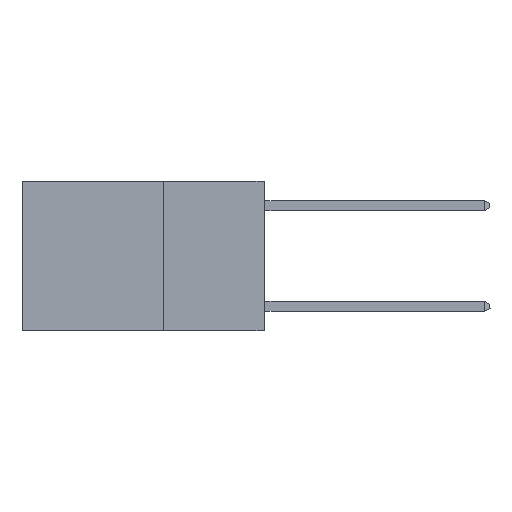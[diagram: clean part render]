
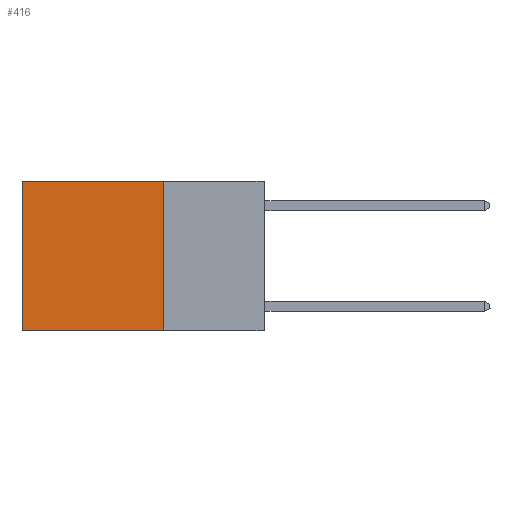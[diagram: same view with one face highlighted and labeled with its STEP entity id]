
A CAD part, left-side view. The second image highlights one B-rep face of the part: STEP entity #416.
In plain terms, the highlighted planar face has unit normal (-1, 0, 0).
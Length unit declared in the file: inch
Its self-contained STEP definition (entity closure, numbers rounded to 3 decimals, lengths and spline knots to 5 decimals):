
#66 = DIRECTION ( 'NONE',  ( 0., 0., -1. ) ) ;
#416 = ADVANCED_FACE ( 'NONE', ( #14020 ), #15484, .F. ) ;
#1102 = CARTESIAN_POINT ( 'NONE',  ( 0.2625, 0.25, 0. ) ) ;
#1451 = AXIS2_PLACEMENT_3D ( 'NONE', #5448, #2985, #66 ) ;
#1620 = VECTOR ( 'NONE', #13045, 39.37008 ) ;
#1746 = CARTESIAN_POINT ( 'NONE',  ( 0.2625, 0.25, 0. ) ) ;
#2985 = DIRECTION ( 'NONE',  ( 1., 0., 0. ) ) ;
#3049 = EDGE_CURVE ( 'NONE', #6684, #14004, #4561, .T. ) ;
#3192 = DIRECTION ( 'NONE',  ( 0., 0., -1. ) ) ;
#4080 = ORIENTED_EDGE ( 'NONE', *, *, #10036, .F. ) ;
#4311 = EDGE_CURVE ( 'NONE', #9819, #14004, #5846, .T. ) ;
#4561 = LINE ( 'NONE', #15691, #16909 ) ;
#5448 = CARTESIAN_POINT ( 'NONE',  ( 0.2625, 0.25, 0. ) ) ;
#5846 = LINE ( 'NONE', #8666, #1620 ) ;
#6370 = ORIENTED_EDGE ( 'NONE', *, *, #12868, .T. ) ;
#6684 = VERTEX_POINT ( 'NONE', #15562 ) ;
#7191 = DIRECTION ( 'NONE',  ( 0., 0., -1. ) ) ;
#8666 = CARTESIAN_POINT ( 'NONE',  ( 0.2625, 0.25, -0.37 ) ) ;
#9568 = CARTESIAN_POINT ( 'NONE',  ( 0.2625, 0.25, -0.37 ) ) ;
#9603 = CARTESIAN_POINT ( 'NONE',  ( 0.2625, 0.25, 0. ) ) ;
#9819 = VERTEX_POINT ( 'NONE', #9568 ) ;
#10022 = EDGE_LOOP ( 'NONE', ( #14485, #12295, #4080, #6370 ) ) ;
#10036 = EDGE_CURVE ( 'NONE', #17938, #9819, #14217, .T. ) ;
#10082 = VECTOR ( 'NONE', #7191, 39.37008 ) ;
#10630 = DIRECTION ( 'NONE',  ( 0., 1., 0. ) ) ;
#12295 = ORIENTED_EDGE ( 'NONE', *, *, #4311, .F. ) ;
#12868 = EDGE_CURVE ( 'NONE', #17938, #6684, #16550, .T. ) ;
#13045 = DIRECTION ( 'NONE',  ( 0., 1., 0. ) ) ;
#13372 = CARTESIAN_POINT ( 'NONE',  ( 0.2625, 0.6, -0.37 ) ) ;
#14004 = VERTEX_POINT ( 'NONE', #13372 ) ;
#14020 = FACE_OUTER_BOUND ( 'NONE', #10022, .T. ) ;
#14217 = LINE ( 'NONE', #1746, #10082 ) ;
#14479 = VECTOR ( 'NONE', #10630, 39.37008 ) ;
#14485 = ORIENTED_EDGE ( 'NONE', *, *, #3049, .T. ) ;
#15484 = PLANE ( 'NONE',  #1451 ) ;
#15562 = CARTESIAN_POINT ( 'NONE',  ( 0.2625, 0.6, 0. ) ) ;
#15691 = CARTESIAN_POINT ( 'NONE',  ( 0.2625, 0.6, 0. ) ) ;
#16550 = LINE ( 'NONE', #9603, #14479 ) ;
#16909 = VECTOR ( 'NONE', #3192, 39.37008 ) ;
#17938 = VERTEX_POINT ( 'NONE', #1102 ) ;
